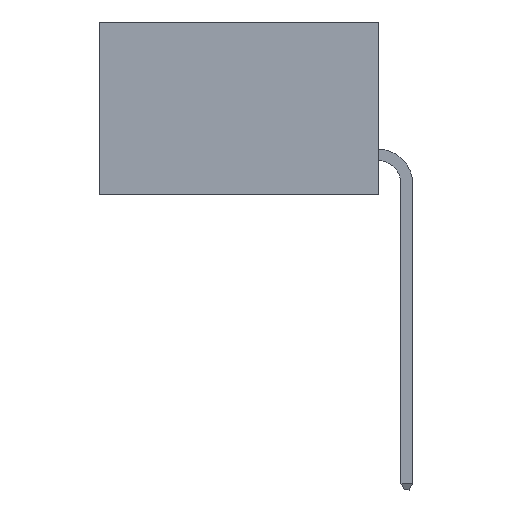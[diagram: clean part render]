
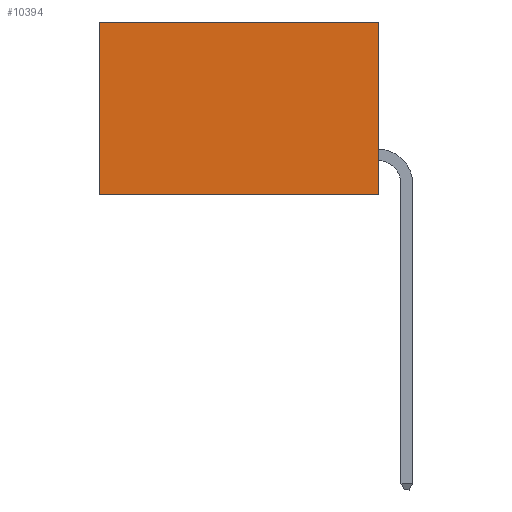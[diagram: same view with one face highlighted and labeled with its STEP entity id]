
A CAD part, left-side view. The second image highlights one B-rep face of the part: STEP entity #10394.
In plain terms, the highlighted planar face has unit normal (-1, 0, 0).
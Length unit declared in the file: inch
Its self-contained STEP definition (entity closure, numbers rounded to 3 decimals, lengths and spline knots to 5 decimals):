
#540 = VERTEX_POINT ( 'NONE', #19916 ) ;
#1358 = CARTESIAN_POINT ( 'NONE',  ( 0.2615, 0., -0.37 ) ) ;
#3322 = ORIENTED_EDGE ( 'NONE', *, *, #13004, .T. ) ;
#3417 = ORIENTED_EDGE ( 'NONE', *, *, #7038, .F. ) ;
#3840 = DIRECTION ( 'NONE',  ( 0., 0., -1. ) ) ;
#5462 = ORIENTED_EDGE ( 'NONE', *, *, #6195, .T. ) ;
#5838 = VERTEX_POINT ( 'NONE', #12230 ) ;
#5908 = LINE ( 'NONE', #7244, #6813 ) ;
#6195 = EDGE_CURVE ( 'NONE', #540, #7708, #13039, .T. ) ;
#6813 = VECTOR ( 'NONE', #13338, 39.37008 ) ;
#6923 = FACE_OUTER_BOUND ( 'NONE', #14994, .T. ) ;
#7038 = EDGE_CURVE ( 'NONE', #540, #5838, #20146, .T. ) ;
#7244 = CARTESIAN_POINT ( 'NONE',  ( 0.2615, 0.6, -0.37 ) ) ;
#7388 = DIRECTION ( 'NONE',  ( 0., 0., -1. ) ) ;
#7708 = VERTEX_POINT ( 'NONE', #17041 ) ;
#8315 = ORIENTED_EDGE ( 'NONE', *, *, #8838, .F. ) ;
#8838 = EDGE_CURVE ( 'NONE', #5838, #12724, #17070, .T. ) ;
#9024 = AXIS2_PLACEMENT_3D ( 'NONE', #11591, #9032, #3840 ) ;
#9032 = DIRECTION ( 'NONE',  ( 1., 0., 0. ) ) ;
#9114 = CARTESIAN_POINT ( 'NONE',  ( 0.2615, 0., -0.37 ) ) ;
#9700 = DIRECTION ( 'NONE',  ( 0., 1., 0. ) ) ;
#10394 = ADVANCED_FACE ( 'NONE', ( #6923 ), #13127, .F. ) ;
#11591 = CARTESIAN_POINT ( 'NONE',  ( 0.2615, 0., -0.37 ) ) ;
#12230 = CARTESIAN_POINT ( 'NONE',  ( 0.2615, 0., -0.37 ) ) ;
#12724 = VERTEX_POINT ( 'NONE', #16938 ) ;
#13004 = EDGE_CURVE ( 'NONE', #7708, #12724, #5908, .T. ) ;
#13039 = LINE ( 'NONE', #19306, #16068 ) ;
#13127 = PLANE ( 'NONE',  #9024 ) ;
#13338 = DIRECTION ( 'NONE',  ( 0., 0., -1. ) ) ;
#14509 = VECTOR ( 'NONE', #7388, 39.37008 ) ;
#14994 = EDGE_LOOP ( 'NONE', ( #3322, #8315, #3417, #5462 ) ) ;
#15939 = VECTOR ( 'NONE', #9700, 39.37008 ) ;
#16068 = VECTOR ( 'NONE', #17771, 39.37008 ) ;
#16938 = CARTESIAN_POINT ( 'NONE',  ( 0.2615, 0.6, -0.37 ) ) ;
#17041 = CARTESIAN_POINT ( 'NONE',  ( 0.2615, 0.6, 0. ) ) ;
#17070 = LINE ( 'NONE', #1358, #15939 ) ;
#17771 = DIRECTION ( 'NONE',  ( 0., 1., 0. ) ) ;
#19306 = CARTESIAN_POINT ( 'NONE',  ( 0.2615, 0., 0. ) ) ;
#19916 = CARTESIAN_POINT ( 'NONE',  ( 0.2615, 0., 0. ) ) ;
#20146 = LINE ( 'NONE', #9114, #14509 ) ;
